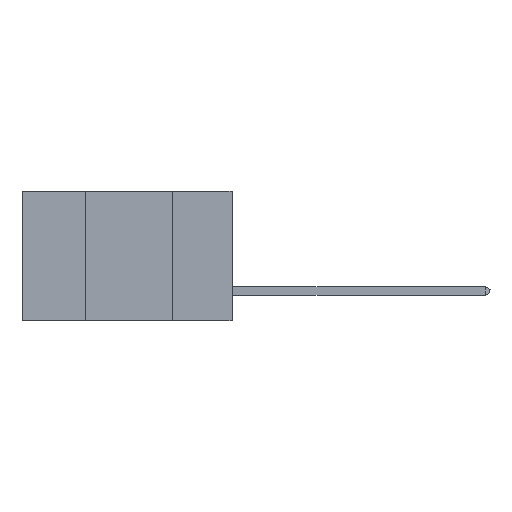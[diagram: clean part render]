
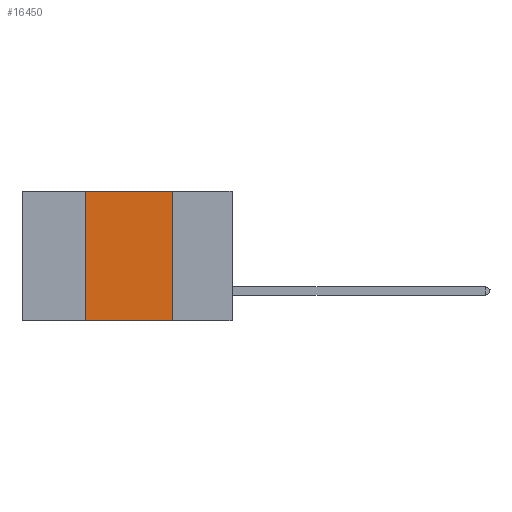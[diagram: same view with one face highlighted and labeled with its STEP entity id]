
A CAD part, left-side view. The second image highlights one B-rep face of the part: STEP entity #16450.
In plain terms, the highlighted planar face has unit normal (-1, 0, 0).
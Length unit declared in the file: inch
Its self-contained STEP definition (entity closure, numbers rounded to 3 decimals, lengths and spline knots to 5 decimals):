
#1155 = CARTESIAN_POINT ( 'NONE',  ( 0., 0.6, -0.37 ) ) ;
#1409 = CARTESIAN_POINT ( 'NONE',  ( 0., 0.17, 0. ) ) ;
#2188 = FACE_OUTER_BOUND ( 'NONE', #6911, .T. ) ;
#2272 = DIRECTION ( 'NONE',  ( 0., 0., -1. ) ) ;
#2694 = AXIS2_PLACEMENT_3D ( 'NONE', #21348, #27898, #41147 ) ;
#2835 = ORIENTED_EDGE ( 'NONE', *, *, #37939, .F. ) ;
#3520 = CARTESIAN_POINT ( 'NONE',  ( 0., 0.17, -0.37 ) ) ;
#4487 = DIRECTION ( 'NONE',  ( 0., 0., 1. ) ) ;
#5192 = LINE ( 'NONE', #1155, #40794 ) ;
#5475 = PLANE ( 'NONE',  #2694 ) ;
#5521 = EDGE_CURVE ( 'NONE', #14262, #24698, #39134, .T. ) ;
#6911 = EDGE_LOOP ( 'NONE', ( #7215, #2835, #41723, #17154 ) ) ;
#7082 = VECTOR ( 'NONE', #4487, 39.37008 ) ;
#7215 = ORIENTED_EDGE ( 'NONE', *, *, #22999, .F. ) ;
#7589 = VECTOR ( 'NONE', #2272, 39.37008 ) ;
#13374 = VECTOR ( 'NONE', #13397, 39.37008 ) ;
#13397 = DIRECTION ( 'NONE',  ( 0., -1., 0. ) ) ;
#14262 = VERTEX_POINT ( 'NONE', #18274 ) ;
#16450 = ADVANCED_FACE ( 'NONE', ( #2188 ), #5475, .F. ) ;
#17154 = ORIENTED_EDGE ( 'NONE', *, *, #36484, .T. ) ;
#17348 = VERTEX_POINT ( 'NONE', #29333 ) ;
#18274 = CARTESIAN_POINT ( 'NONE',  ( 0., 0.42, -0.37 ) ) ;
#18815 = CARTESIAN_POINT ( 'NONE',  ( 0., 0.42, 0. ) ) ;
#21211 = VERTEX_POINT ( 'NONE', #3520 ) ;
#21348 = CARTESIAN_POINT ( 'NONE',  ( 0., 0.6, 0. ) ) ;
#22999 = EDGE_CURVE ( 'NONE', #17348, #21211, #29929, .T. ) ;
#23658 = DIRECTION ( 'NONE',  ( 0., -1., 0. ) ) ;
#24698 = VERTEX_POINT ( 'NONE', #18815 ) ;
#27898 = DIRECTION ( 'NONE',  ( 1., 0., 0. ) ) ;
#29333 = CARTESIAN_POINT ( 'NONE',  ( 0., 0.17, 0. ) ) ;
#29929 = LINE ( 'NONE', #1409, #7589 ) ;
#32109 = LINE ( 'NONE', #39344, #13374 ) ;
#36484 = EDGE_CURVE ( 'NONE', #14262, #21211, #5192, .T. ) ;
#37939 = EDGE_CURVE ( 'NONE', #24698, #17348, #32109, .T. ) ;
#39134 = LINE ( 'NONE', #40308, #7082 ) ;
#39344 = CARTESIAN_POINT ( 'NONE',  ( 0., 0.6, 0. ) ) ;
#40308 = CARTESIAN_POINT ( 'NONE',  ( 0., 0.42, 0. ) ) ;
#40794 = VECTOR ( 'NONE', #23658, 39.37008 ) ;
#41147 = DIRECTION ( 'NONE',  ( 0., 0., -1. ) ) ;
#41723 = ORIENTED_EDGE ( 'NONE', *, *, #5521, .F. ) ;
